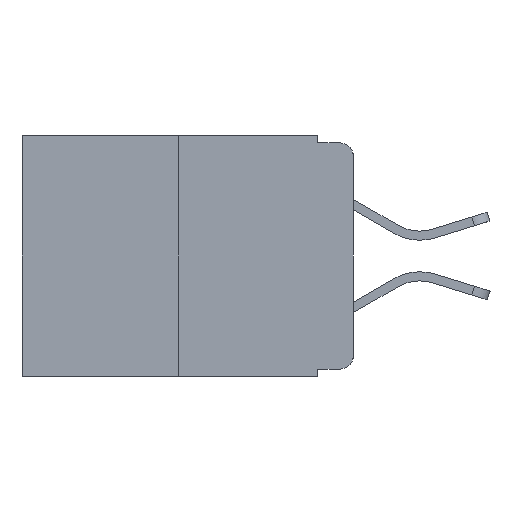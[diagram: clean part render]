
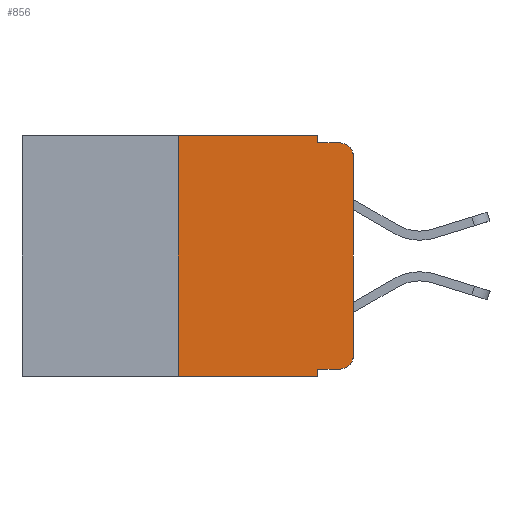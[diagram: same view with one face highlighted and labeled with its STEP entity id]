
A CAD part, left-side view. The second image highlights one B-rep face of the part: STEP entity #856.
In plain terms, the highlighted planar face has unit normal (-1, 0, 0).
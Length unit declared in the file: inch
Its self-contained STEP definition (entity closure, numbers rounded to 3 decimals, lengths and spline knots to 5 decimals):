
#17 = VERTEX_POINT ( 'NONE', #11101 ) ;
#39 = VERTEX_POINT ( 'NONE', #499 ) ;
#76 = CARTESIAN_POINT ( 'NONE',  ( 0., 0.051, -0.333 ) ) ;
#122 = LINE ( 'NONE', #11896, #2143 ) ;
#499 = CARTESIAN_POINT ( 'NONE',  ( 0., 0.051, -0.01 ) ) ;
#530 = ORIENTED_EDGE ( 'NONE', *, *, #7320, .F. ) ;
#546 = LINE ( 'NONE', #11149, #10477 ) ;
#603 = DIRECTION ( 'NONE',  ( 0., 0., -1. ) ) ;
#616 = VERTEX_POINT ( 'NONE', #11831 ) ;
#619 = VERTEX_POINT ( 'NONE', #11703 ) ;
#710 = ORIENTED_EDGE ( 'NONE', *, *, #3916, .T. ) ;
#847 = ORIENTED_EDGE ( 'NONE', *, *, #7527, .F. ) ;
#852 = EDGE_CURVE ( 'NONE', #10688, #619, #4899, .T. ) ;
#856 = ADVANCED_FACE ( 'NONE', ( #9048 ), #7230, .F. ) ;
#1135 = DIRECTION ( 'NONE',  ( 0., 0., 1. ) ) ;
#1401 = CARTESIAN_POINT ( 'NONE',  ( 0., 0.051, 0. ) ) ;
#1444 = VERTEX_POINT ( 'NONE', #7199 ) ;
#1491 = AXIS2_PLACEMENT_3D ( 'NONE', #13306, #7096, #3830 ) ;
#1635 = DIRECTION ( 'NONE',  ( 0., -1., 0. ) ) ;
#1649 = CARTESIAN_POINT ( 'NONE',  ( 0., 0.25, 0. ) ) ;
#1679 = DIRECTION ( 'NONE',  ( -1., 0., 0. ) ) ;
#1736 = EDGE_CURVE ( 'NONE', #1816, #1444, #546, .T. ) ;
#1816 = VERTEX_POINT ( 'NONE', #5245 ) ;
#2143 = VECTOR ( 'NONE', #8768, 39.37008 ) ;
#2300 = LINE ( 'NONE', #4519, #7784 ) ;
#2597 = VECTOR ( 'NONE', #1135, 39.37008 ) ;
#2672 = DIRECTION ( 'NONE',  ( -1., 0., 0. ) ) ;
#2676 = AXIS2_PLACEMENT_3D ( 'NONE', #10103, #2672, #603 ) ;
#2911 = VECTOR ( 'NONE', #13147, 39.37008 ) ;
#3562 = EDGE_LOOP ( 'NONE', ( #11714, #6677, #847, #6696, #530, #9756, #8823, #12440, #710, #10294 ) ) ;
#3767 = DIRECTION ( 'NONE',  ( 0., -1., 0. ) ) ;
#3794 = VERTEX_POINT ( 'NONE', #1649 ) ;
#3830 = DIRECTION ( 'NONE',  ( 0., 0., -1. ) ) ;
#3885 = CARTESIAN_POINT ( 'NONE',  ( 0., 0.02, -0.333 ) ) ;
#3916 = EDGE_CURVE ( 'NONE', #616, #10688, #6221, .T. ) ;
#4308 = LINE ( 'NONE', #10485, #9075 ) ;
#4519 = CARTESIAN_POINT ( 'NONE',  ( 0., 0.25, 0. ) ) ;
#4791 = EDGE_CURVE ( 'NONE', #17, #39, #4308, .T. ) ;
#4899 = CIRCLE ( 'NONE', #9346, 0.02 ) ;
#5245 = CARTESIAN_POINT ( 'NONE',  ( 0., 0.25, -0.343 ) ) ;
#5492 = DIRECTION ( 'NONE',  ( 0., 0., 1. ) ) ;
#5616 = CARTESIAN_POINT ( 'NONE',  ( 0., 0., 0. ) ) ;
#5833 = VERTEX_POINT ( 'NONE', #9410 ) ;
#6221 = LINE ( 'NONE', #76, #8350 ) ;
#6296 = DIRECTION ( 'NONE',  ( 0., -1., 0. ) ) ;
#6677 = ORIENTED_EDGE ( 'NONE', *, *, #9975, .T. ) ;
#6696 = ORIENTED_EDGE ( 'NONE', *, *, #4791, .F. ) ;
#7096 = DIRECTION ( 'NONE',  ( 1., 0., 0. ) ) ;
#7199 = CARTESIAN_POINT ( 'NONE',  ( 0., 0.051, -0.343 ) ) ;
#7230 = PLANE ( 'NONE',  #1491 ) ;
#7320 = EDGE_CURVE ( 'NONE', #3794, #17, #122, .T. ) ;
#7499 = LINE ( 'NONE', #5616, #2597 ) ;
#7527 = EDGE_CURVE ( 'NONE', #39, #11519, #11277, .T. ) ;
#7784 = VECTOR ( 'NONE', #5492, 39.37008 ) ;
#7983 = CARTESIAN_POINT ( 'NONE',  ( 0., 0.02, -0.01 ) ) ;
#8350 = VECTOR ( 'NONE', #6296, 39.37008 ) ;
#8468 = DIRECTION ( 'NONE',  ( 0., 0., -1. ) ) ;
#8768 = DIRECTION ( 'NONE',  ( 0., -1., 0. ) ) ;
#8823 = ORIENTED_EDGE ( 'NONE', *, *, #1736, .T. ) ;
#9035 = EDGE_CURVE ( 'NONE', #616, #1444, #12941, .T. ) ;
#9048 = FACE_OUTER_BOUND ( 'NONE', #3562, .T. ) ;
#9075 = VECTOR ( 'NONE', #8468, 39.37008 ) ;
#9346 = AXIS2_PLACEMENT_3D ( 'NONE', #12245, #1679, #12102 ) ;
#9410 = CARTESIAN_POINT ( 'NONE',  ( 0., 0., -0.03 ) ) ;
#9756 = ORIENTED_EDGE ( 'NONE', *, *, #12149, .F. ) ;
#9975 = EDGE_CURVE ( 'NONE', #5833, #11519, #13239, .T. ) ;
#10103 = CARTESIAN_POINT ( 'NONE',  ( 0., 0.02, -0.03 ) ) ;
#10294 = ORIENTED_EDGE ( 'NONE', *, *, #852, .T. ) ;
#10477 = VECTOR ( 'NONE', #1635, 39.37008 ) ;
#10485 = CARTESIAN_POINT ( 'NONE',  ( 0., 0.051, 0. ) ) ;
#10688 = VERTEX_POINT ( 'NONE', #3885 ) ;
#11101 = CARTESIAN_POINT ( 'NONE',  ( 0., 0.051, 0. ) ) ;
#11149 = CARTESIAN_POINT ( 'NONE',  ( 0., 0.473, -0.343 ) ) ;
#11277 = LINE ( 'NONE', #13166, #11901 ) ;
#11519 = VERTEX_POINT ( 'NONE', #7983 ) ;
#11703 = CARTESIAN_POINT ( 'NONE',  ( 0., 0., -0.313 ) ) ;
#11714 = ORIENTED_EDGE ( 'NONE', *, *, #12613, .T. ) ;
#11831 = CARTESIAN_POINT ( 'NONE',  ( 0., 0.051, -0.333 ) ) ;
#11896 = CARTESIAN_POINT ( 'NONE',  ( 0., 0.473, 0. ) ) ;
#11901 = VECTOR ( 'NONE', #3767, 39.37008 ) ;
#12102 = DIRECTION ( 'NONE',  ( 0., 0., -1. ) ) ;
#12149 = EDGE_CURVE ( 'NONE', #1816, #3794, #2300, .T. ) ;
#12245 = CARTESIAN_POINT ( 'NONE',  ( 0., 0.02, -0.313 ) ) ;
#12440 = ORIENTED_EDGE ( 'NONE', *, *, #9035, .F. ) ;
#12613 = EDGE_CURVE ( 'NONE', #619, #5833, #7499, .T. ) ;
#12941 = LINE ( 'NONE', #1401, #2911 ) ;
#13147 = DIRECTION ( 'NONE',  ( 0., 0., -1. ) ) ;
#13166 = CARTESIAN_POINT ( 'NONE',  ( 0., 0.051, -0.01 ) ) ;
#13239 = CIRCLE ( 'NONE', #2676, 0.02 ) ;
#13306 = CARTESIAN_POINT ( 'NONE',  ( 0., 0.473, 0. ) ) ;
